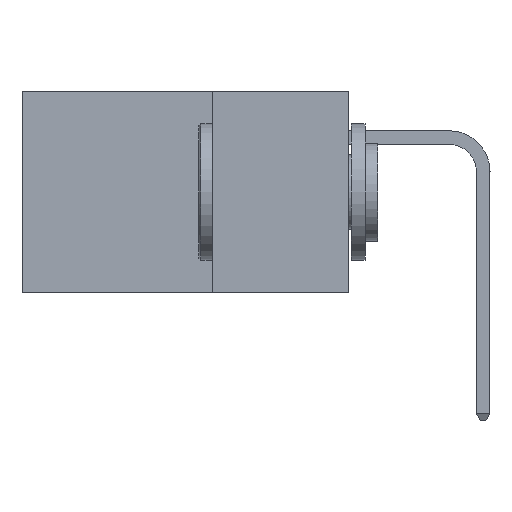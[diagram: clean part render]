
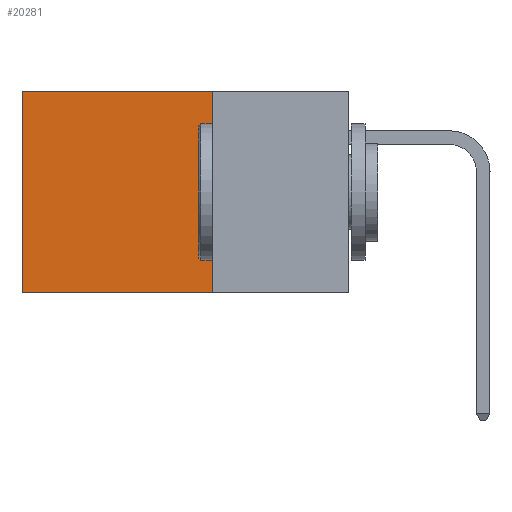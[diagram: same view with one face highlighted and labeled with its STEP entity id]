
A CAD part, left-side view. The second image highlights one B-rep face of the part: STEP entity #20281.
In plain terms, the highlighted planar face has unit normal (-1, 0, 0).
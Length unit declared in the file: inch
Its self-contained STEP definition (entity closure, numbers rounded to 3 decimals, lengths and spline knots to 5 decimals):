
#589 = VECTOR ( 'NONE', #3954, 39.37008 ) ;
#753 = VERTEX_POINT ( 'NONE', #14271 ) ;
#902 = EDGE_LOOP ( 'NONE', ( #8922, #3495, #6522, #2816 ) ) ;
#2816 = ORIENTED_EDGE ( 'NONE', *, *, #11091, .T. ) ;
#2892 = LINE ( 'NONE', #3945, #17638 ) ;
#3495 = ORIENTED_EDGE ( 'NONE', *, *, #9195, .F. ) ;
#3945 = CARTESIAN_POINT ( 'NONE',  ( 0.2875, 0.25, -0.37 ) ) ;
#3954 = DIRECTION ( 'NONE',  ( 0., 0., -1. ) ) ;
#4393 = AXIS2_PLACEMENT_3D ( 'NONE', #4456, #10426, #12331 ) ;
#4456 = CARTESIAN_POINT ( 'NONE',  ( 0.2875, 0.25, 0. ) ) ;
#5765 = VERTEX_POINT ( 'NONE', #6638 ) ;
#6522 = ORIENTED_EDGE ( 'NONE', *, *, #12992, .F. ) ;
#6638 = CARTESIAN_POINT ( 'NONE',  ( 0.2875, 0.25, -0.37 ) ) ;
#6864 = CARTESIAN_POINT ( 'NONE',  ( 0.2875, 0.6, 0. ) ) ;
#7343 = VECTOR ( 'NONE', #16581, 39.37008 ) ;
#8468 = LINE ( 'NONE', #9689, #589 ) ;
#8566 = CARTESIAN_POINT ( 'NONE',  ( 0.2875, 0.25, 0. ) ) ;
#8922 = ORIENTED_EDGE ( 'NONE', *, *, #20891, .T. ) ;
#9195 = EDGE_CURVE ( 'NONE', #5765, #753, #2892, .T. ) ;
#9329 = VERTEX_POINT ( 'NONE', #8566 ) ;
#9689 = CARTESIAN_POINT ( 'NONE',  ( 0.2875, 0.25, 0. ) ) ;
#10426 = DIRECTION ( 'NONE',  ( 1., 0., 0. ) ) ;
#11091 = EDGE_CURVE ( 'NONE', #9329, #12328, #13349, .T. ) ;
#12328 = VERTEX_POINT ( 'NONE', #17173 ) ;
#12331 = DIRECTION ( 'NONE',  ( 0., 0., -1. ) ) ;
#12742 = VECTOR ( 'NONE', #21764, 39.37008 ) ;
#12992 = EDGE_CURVE ( 'NONE', #9329, #5765, #8468, .T. ) ;
#13349 = LINE ( 'NONE', #21851, #12742 ) ;
#14271 = CARTESIAN_POINT ( 'NONE',  ( 0.2875, 0.6, -0.37 ) ) ;
#16581 = DIRECTION ( 'NONE',  ( 0., 0., -1. ) ) ;
#17173 = CARTESIAN_POINT ( 'NONE',  ( 0.2875, 0.6, 0. ) ) ;
#17391 = DIRECTION ( 'NONE',  ( 0., 1., 0. ) ) ;
#17638 = VECTOR ( 'NONE', #17391, 39.37008 ) ;
#19362 = LINE ( 'NONE', #6864, #7343 ) ;
#19717 = PLANE ( 'NONE',  #4393 ) ;
#20281 = ADVANCED_FACE ( 'NONE', ( #22976 ), #19717, .F. ) ;
#20891 = EDGE_CURVE ( 'NONE', #12328, #753, #19362, .T. ) ;
#21764 = DIRECTION ( 'NONE',  ( 0., 1., 0. ) ) ;
#21851 = CARTESIAN_POINT ( 'NONE',  ( 0.2875, 0.25, 0. ) ) ;
#22976 = FACE_OUTER_BOUND ( 'NONE', #902, .T. ) ;
